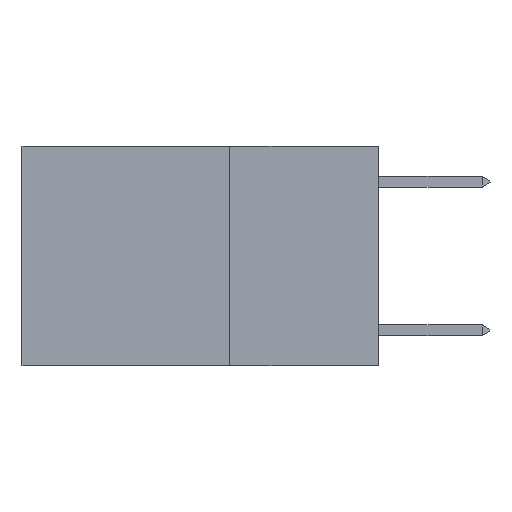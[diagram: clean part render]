
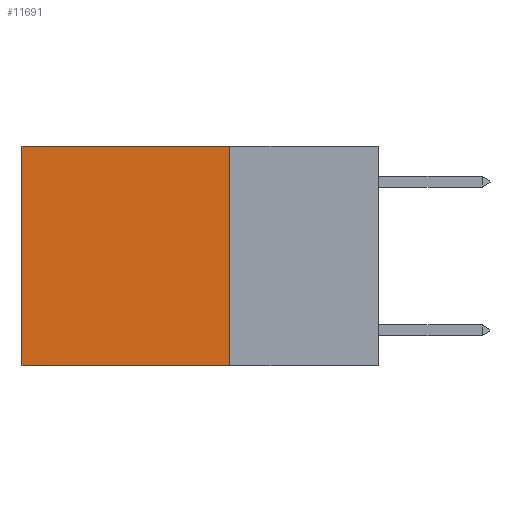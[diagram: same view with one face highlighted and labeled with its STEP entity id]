
A CAD part, left-side view. The second image highlights one B-rep face of the part: STEP entity #11691.
In plain terms, the highlighted planar face has unit normal (-1, 0, 0).
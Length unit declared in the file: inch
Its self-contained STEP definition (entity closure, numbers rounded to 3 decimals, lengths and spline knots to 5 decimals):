
#117 = CARTESIAN_POINT ( 'NONE',  ( 0.2625, 0.25, 0. ) ) ;
#187 = LINE ( 'NONE', #12998, #17527 ) ;
#680 = LINE ( 'NONE', #117, #7735 ) ;
#843 = CARTESIAN_POINT ( 'NONE',  ( 0.2625, 0.25, -0.37 ) ) ;
#942 = AXIS2_PLACEMENT_3D ( 'NONE', #4148, #13798, #5564 ) ;
#1554 = VERTEX_POINT ( 'NONE', #1922 ) ;
#1623 = LINE ( 'NONE', #843, #15827 ) ;
#1922 = CARTESIAN_POINT ( 'NONE',  ( 0.2625, 0.6, -0.37 ) ) ;
#1980 = CARTESIAN_POINT ( 'NONE',  ( 0.2625, 0.25, -0.37 ) ) ;
#2164 = ORIENTED_EDGE ( 'NONE', *, *, #5341, .F. ) ;
#2698 = CARTESIAN_POINT ( 'NONE',  ( 0.2625, 0.6, 0. ) ) ;
#4148 = CARTESIAN_POINT ( 'NONE',  ( 0.2625, 0.25, 0. ) ) ;
#5341 = EDGE_CURVE ( 'NONE', #9998, #1554, #1623, .T. ) ;
#5564 = DIRECTION ( 'NONE',  ( 0., 0., -1. ) ) ;
#5571 = VECTOR ( 'NONE', #10050, 39.37008 ) ;
#5782 = EDGE_LOOP ( 'NONE', ( #15427, #2164, #11856, #15085 ) ) ;
#5824 = CARTESIAN_POINT ( 'NONE',  ( 0.2625, 0.25, 0. ) ) ;
#5884 = VERTEX_POINT ( 'NONE', #10284 ) ;
#6531 = EDGE_CURVE ( 'NONE', #5884, #10960, #680, .T. ) ;
#7581 = DIRECTION ( 'NONE',  ( 0., 0., -1. ) ) ;
#7735 = VECTOR ( 'NONE', #13951, 39.37008 ) ;
#8698 = EDGE_CURVE ( 'NONE', #10960, #1554, #187, .T. ) ;
#9998 = VERTEX_POINT ( 'NONE', #1980 ) ;
#10050 = DIRECTION ( 'NONE',  ( 0., 0., -1. ) ) ;
#10284 = CARTESIAN_POINT ( 'NONE',  ( 0.2625, 0.25, 0. ) ) ;
#10960 = VERTEX_POINT ( 'NONE', #2698 ) ;
#11466 = FACE_OUTER_BOUND ( 'NONE', #5782, .T. ) ;
#11691 = ADVANCED_FACE ( 'NONE', ( #11466 ), #13747, .F. ) ;
#11856 = ORIENTED_EDGE ( 'NONE', *, *, #16330, .F. ) ;
#12998 = CARTESIAN_POINT ( 'NONE',  ( 0.2625, 0.6, 0. ) ) ;
#13339 = DIRECTION ( 'NONE',  ( 0., 1., 0. ) ) ;
#13747 = PLANE ( 'NONE',  #942 ) ;
#13798 = DIRECTION ( 'NONE',  ( 1., 0., 0. ) ) ;
#13951 = DIRECTION ( 'NONE',  ( 0., 1., 0. ) ) ;
#15085 = ORIENTED_EDGE ( 'NONE', *, *, #6531, .T. ) ;
#15427 = ORIENTED_EDGE ( 'NONE', *, *, #8698, .T. ) ;
#15827 = VECTOR ( 'NONE', #13339, 39.37008 ) ;
#16330 = EDGE_CURVE ( 'NONE', #5884, #9998, #16422, .T. ) ;
#16422 = LINE ( 'NONE', #5824, #5571 ) ;
#17527 = VECTOR ( 'NONE', #7581, 39.37008 ) ;
